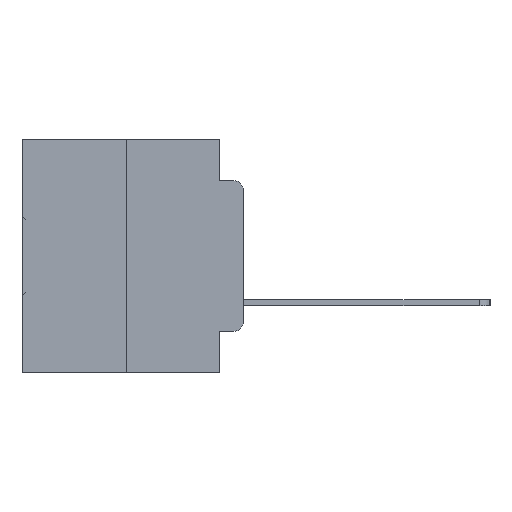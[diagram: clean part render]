
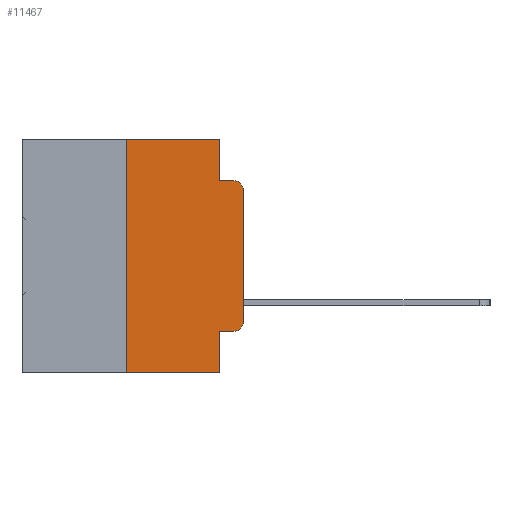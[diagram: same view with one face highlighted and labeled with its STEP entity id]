
A CAD part, left-side view. The second image highlights one B-rep face of the part: STEP entity #11467.
In plain terms, the highlighted planar face has unit normal (-1, 0, 0).
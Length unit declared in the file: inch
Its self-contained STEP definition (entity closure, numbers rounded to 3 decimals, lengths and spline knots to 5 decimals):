
#132 = AXIS2_PLACEMENT_3D ( 'NONE', #26390, #29134, #12769 ) ;
#836 = DIRECTION ( 'NONE',  ( 0., -1., 0. ) ) ;
#884 = CARTESIAN_POINT ( 'NONE',  ( 0., 0.02, -0.3915 ) ) ;
#1525 = ORIENTED_EDGE ( 'NONE', *, *, #5833, .T. ) ;
#1642 = PLANE ( 'NONE',  #132 ) ;
#1897 = CARTESIAN_POINT ( 'NONE',  ( 0., 0.051, -0.0885 ) ) ;
#2009 = DIRECTION ( 'NONE',  ( 0., 0., 1. ) ) ;
#2655 = CARTESIAN_POINT ( 'NONE',  ( 0., 0.25, -0.5 ) ) ;
#3679 = DIRECTION ( 'NONE',  ( 0., 0., -1. ) ) ;
#3805 = DIRECTION ( 'NONE',  ( 0., -1., 0. ) ) ;
#5161 = EDGE_CURVE ( 'NONE', #33137, #11726, #26070, .T. ) ;
#5833 = EDGE_CURVE ( 'NONE', #20394, #33137, #10186, .T. ) ;
#6004 = LINE ( 'NONE', #20282, #19789 ) ;
#6078 = VERTEX_POINT ( 'NONE', #7526 ) ;
#6255 = CARTESIAN_POINT ( 'NONE',  ( 0., 0.25, 0. ) ) ;
#7526 = CARTESIAN_POINT ( 'NONE',  ( 0., 0.02, -0.0885 ) ) ;
#8001 = EDGE_LOOP ( 'NONE', ( #19179, #24318, #11483, #33176, #30272, #31099, #10197, #11914, #8041, #1525 ) ) ;
#8041 = ORIENTED_EDGE ( 'NONE', *, *, #15076, .T. ) ;
#8469 = VERTEX_POINT ( 'NONE', #2655 ) ;
#8925 = VECTOR ( 'NONE', #836, 39.37008 ) ;
#9350 = EDGE_CURVE ( 'NONE', #8469, #14952, #6004, .T. ) ;
#10186 = CIRCLE ( 'NONE', #27878, 0.02 ) ;
#10197 = ORIENTED_EDGE ( 'NONE', *, *, #9350, .T. ) ;
#10270 = DIRECTION ( 'NONE',  ( 0., -1., 0. ) ) ;
#11099 = LINE ( 'NONE', #1897, #31966 ) ;
#11467 = ADVANCED_FACE ( 'NONE', ( #12879 ), #1642, .F. ) ;
#11483 = ORIENTED_EDGE ( 'NONE', *, *, #27897, .F. ) ;
#11534 = DIRECTION ( 'NONE',  ( 0., 0., -1. ) ) ;
#11726 = VERTEX_POINT ( 'NONE', #30286 ) ;
#11824 = CARTESIAN_POINT ( 'NONE',  ( 0., 0., 0. ) ) ;
#11914 = ORIENTED_EDGE ( 'NONE', *, *, #16906, .F. ) ;
#11929 = VERTEX_POINT ( 'NONE', #14767 ) ;
#12294 = CARTESIAN_POINT ( 'NONE',  ( 0., 0.02, -0.4115 ) ) ;
#12449 = VECTOR ( 'NONE', #27310, 39.37008 ) ;
#12769 = DIRECTION ( 'NONE',  ( 0., 0., -1. ) ) ;
#12879 = FACE_OUTER_BOUND ( 'NONE', #8001, .T. ) ;
#13279 = CARTESIAN_POINT ( 'NONE',  ( 0., 0.02, -0.1085 ) ) ;
#13719 = CARTESIAN_POINT ( 'NONE',  ( 0., 0.051, 0. ) ) ;
#13880 = CARTESIAN_POINT ( 'NONE',  ( 0., 0.051, -0.4115 ) ) ;
#13906 = VERTEX_POINT ( 'NONE', #24590 ) ;
#14098 = VECTOR ( 'NONE', #11534, 39.37008 ) ;
#14767 = CARTESIAN_POINT ( 'NONE',  ( 0., 0.051, 0. ) ) ;
#14942 = LINE ( 'NONE', #25157, #14098 ) ;
#14952 = VERTEX_POINT ( 'NONE', #18661 ) ;
#15076 = EDGE_CURVE ( 'NONE', #32689, #20394, #18657, .T. ) ;
#16023 = DIRECTION ( 'NONE',  ( 0., 0., -1. ) ) ;
#16233 = LINE ( 'NONE', #17362, #8925 ) ;
#16896 = CARTESIAN_POINT ( 'NONE',  ( 0., 0., -0.3915 ) ) ;
#16906 = EDGE_CURVE ( 'NONE', #32689, #14952, #14942, .T. ) ;
#17362 = CARTESIAN_POINT ( 'NONE',  ( 0., 0.473, 0. ) ) ;
#17791 = VECTOR ( 'NONE', #2009, 39.37008 ) ;
#18229 = AXIS2_PLACEMENT_3D ( 'NONE', #13279, #32300, #16023 ) ;
#18657 = LINE ( 'NONE', #13880, #25066 ) ;
#18661 = CARTESIAN_POINT ( 'NONE',  ( 0., 0.051, -0.5 ) ) ;
#18747 = EDGE_CURVE ( 'NONE', #8469, #27615, #25070, .T. ) ;
#18816 = VECTOR ( 'NONE', #22860, 39.37008 ) ;
#19179 = ORIENTED_EDGE ( 'NONE', *, *, #5161, .T. ) ;
#19743 = LINE ( 'NONE', #13719, #12449 ) ;
#19789 = VECTOR ( 'NONE', #3805, 39.37008 ) ;
#20176 = DIRECTION ( 'NONE',  ( -1., 0., 0. ) ) ;
#20282 = CARTESIAN_POINT ( 'NONE',  ( 0., 0.473, -0.5 ) ) ;
#20394 = VERTEX_POINT ( 'NONE', #12294 ) ;
#20542 = CARTESIAN_POINT ( 'NONE',  ( 0., 0.051, -0.4115 ) ) ;
#22860 = DIRECTION ( 'NONE',  ( 0., 0., 1. ) ) ;
#24318 = ORIENTED_EDGE ( 'NONE', *, *, #29711, .T. ) ;
#24590 = CARTESIAN_POINT ( 'NONE',  ( 0., 0.051, -0.0885 ) ) ;
#25066 = VECTOR ( 'NONE', #30203, 39.37008 ) ;
#25070 = LINE ( 'NONE', #26633, #17791 ) ;
#25157 = CARTESIAN_POINT ( 'NONE',  ( 0., 0.051, 0. ) ) ;
#26059 = EDGE_CURVE ( 'NONE', #11929, #13906, #19743, .T. ) ;
#26070 = LINE ( 'NONE', #11824, #18816 ) ;
#26390 = CARTESIAN_POINT ( 'NONE',  ( 0., 0.473, 0. ) ) ;
#26633 = CARTESIAN_POINT ( 'NONE',  ( 0., 0.25, 0. ) ) ;
#27310 = DIRECTION ( 'NONE',  ( 0., 0., -1. ) ) ;
#27615 = VERTEX_POINT ( 'NONE', #6255 ) ;
#27878 = AXIS2_PLACEMENT_3D ( 'NONE', #884, #20176, #3679 ) ;
#27897 = EDGE_CURVE ( 'NONE', #13906, #6078, #11099, .T. ) ;
#29099 = CIRCLE ( 'NONE', #18229, 0.02 ) ;
#29134 = DIRECTION ( 'NONE',  ( 1., 0., 0. ) ) ;
#29711 = EDGE_CURVE ( 'NONE', #11726, #6078, #29099, .T. ) ;
#30203 = DIRECTION ( 'NONE',  ( 0., -1., 0. ) ) ;
#30272 = ORIENTED_EDGE ( 'NONE', *, *, #31163, .F. ) ;
#30286 = CARTESIAN_POINT ( 'NONE',  ( 0., 0., -0.1085 ) ) ;
#31099 = ORIENTED_EDGE ( 'NONE', *, *, #18747, .F. ) ;
#31163 = EDGE_CURVE ( 'NONE', #27615, #11929, #16233, .T. ) ;
#31966 = VECTOR ( 'NONE', #10270, 39.37008 ) ;
#32300 = DIRECTION ( 'NONE',  ( -1., 0., 0. ) ) ;
#32689 = VERTEX_POINT ( 'NONE', #20542 ) ;
#33137 = VERTEX_POINT ( 'NONE', #16896 ) ;
#33176 = ORIENTED_EDGE ( 'NONE', *, *, #26059, .F. ) ;
